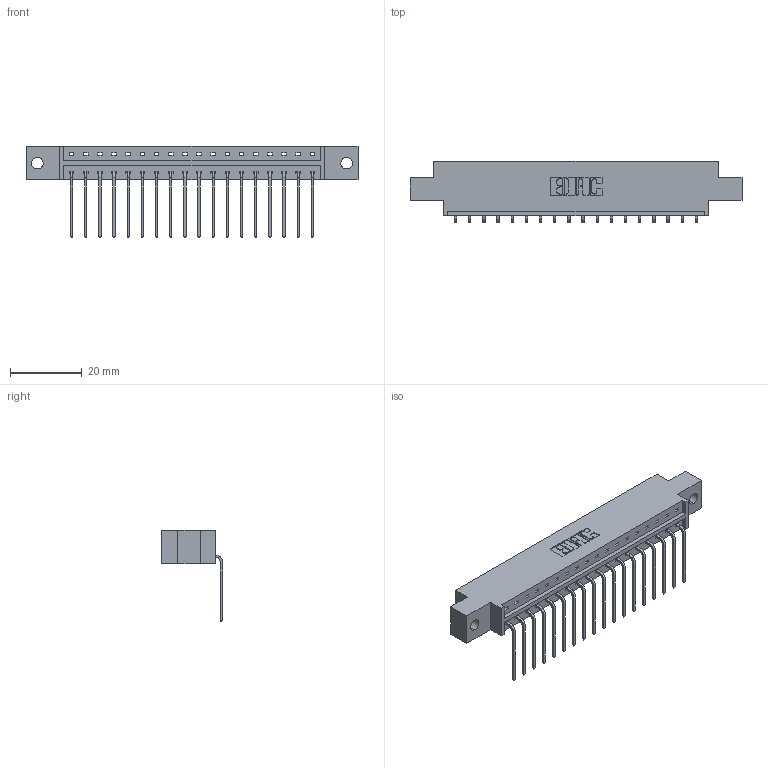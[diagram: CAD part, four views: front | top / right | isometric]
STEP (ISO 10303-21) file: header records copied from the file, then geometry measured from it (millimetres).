
FILE_DESCRIPTION (( 'STEP AP203' ), '1' );
FILE_NAME ('833-018-559-602.STEP', '2020-05-31T23:31:09', ( '' ), ( '' ), 'SwSTEP 2.0', 'SolidWorks 2020', '' );
FILE_SCHEMA (( 'CONFIG_CONTROL_DESIGN' ));
Length unit declared in the file: inch
Products named in the file (3): 345-292-001_558 559 Tail - 1; 833 Part_Offset - .128 Dia; 833-018-559-602
Assembly tree (19 placements, depth 2):
  833-018-559-602
    833 Part_Offset - .128 Dia
    345-292-001_558 559 Tail - 1  x18
Bounding box: 92.86 x 17.09 x 25.53 mm (x, y, z)
Volume: 8933.7 mm3; surface area: 9802.5 mm2
Topology: 19 solids, 19 shells, 1198 faces, 3599 edges, 2374 vertices
Faces by surface type: plane 866, cylinder 332
Entity records: 14327 total; most frequent: CARTESIAN_POINT 2484, ORIENTED_EDGE 2438, DIRECTION 2143, EDGE_CURVE 1219, VECTOR 1091, LINE 1091, VERTEX_POINT 810, AXIS2_PLACEMENT_3D 526
